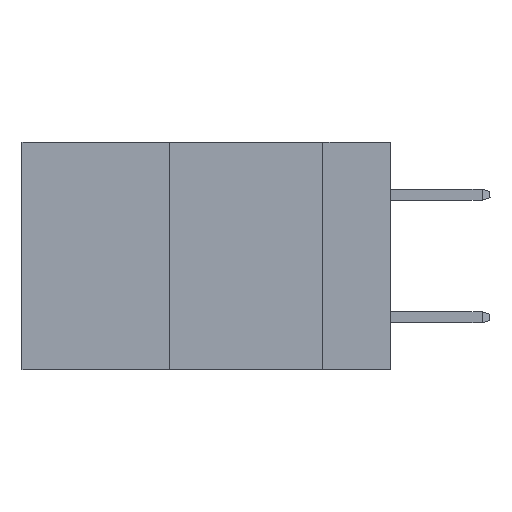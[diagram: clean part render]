
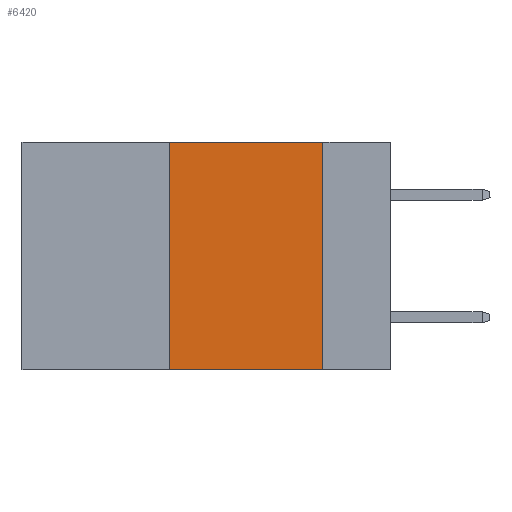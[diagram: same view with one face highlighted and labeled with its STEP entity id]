
A CAD part, left-side view. The second image highlights one B-rep face of the part: STEP entity #6420.
In plain terms, the highlighted planar face has unit normal (-1, 0, 0).
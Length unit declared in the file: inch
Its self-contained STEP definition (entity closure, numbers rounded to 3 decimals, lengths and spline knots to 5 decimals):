
#616 = CARTESIAN_POINT ( 'NONE',  ( 0., 0.6, 0. ) ) ;
#1344 = VECTOR ( 'NONE', #9300, 39.37008 ) ;
#1706 = DIRECTION ( 'NONE',  ( 0., 0., -1. ) ) ;
#1831 = CARTESIAN_POINT ( 'NONE',  ( 0., 0.11, 0. ) ) ;
#1977 = DIRECTION ( 'NONE',  ( 0., 0., -1. ) ) ;
#2207 = EDGE_CURVE ( 'NONE', #10146, #8205, #5850, .T. ) ;
#3096 = EDGE_CURVE ( 'NONE', #8205, #6480, #4719, .T. ) ;
#3157 = ORIENTED_EDGE ( 'NONE', *, *, #2207, .F. ) ;
#4719 = LINE ( 'NONE', #7437, #6367 ) ;
#5142 = ORIENTED_EDGE ( 'NONE', *, *, #13858, .T. ) ;
#5850 = LINE ( 'NONE', #616, #12321 ) ;
#6367 = VECTOR ( 'NONE', #1706, 39.37008 ) ;
#6420 = ADVANCED_FACE ( 'NONE', ( #14247 ), #9976, .F. ) ;
#6480 = VERTEX_POINT ( 'NONE', #14125 ) ;
#7437 = CARTESIAN_POINT ( 'NONE',  ( 0., 0.11, 0. ) ) ;
#8205 = VERTEX_POINT ( 'NONE', #1831 ) ;
#8292 = ORIENTED_EDGE ( 'NONE', *, *, #8927, .F. ) ;
#8363 = CARTESIAN_POINT ( 'NONE',  ( 0., 0.36, 0. ) ) ;
#8927 = EDGE_CURVE ( 'NONE', #10553, #10146, #13798, .T. ) ;
#9061 = EDGE_LOOP ( 'NONE', ( #10033, #3157, #8292, #5142 ) ) ;
#9300 = DIRECTION ( 'NONE',  ( 0., 0., 1. ) ) ;
#9951 = DIRECTION ( 'NONE',  ( 0., -1., 0. ) ) ;
#9976 = PLANE ( 'NONE',  #10563 ) ;
#10033 = ORIENTED_EDGE ( 'NONE', *, *, #3096, .F. ) ;
#10146 = VERTEX_POINT ( 'NONE', #8363 ) ;
#10553 = VERTEX_POINT ( 'NONE', #13657 ) ;
#10563 = AXIS2_PLACEMENT_3D ( 'NONE', #10918, #12286, #1977 ) ;
#10868 = CARTESIAN_POINT ( 'NONE',  ( 0., 0.36, 0. ) ) ;
#10918 = CARTESIAN_POINT ( 'NONE',  ( 0., 0.6, 0. ) ) ;
#11051 = DIRECTION ( 'NONE',  ( 0., -1., 0. ) ) ;
#11470 = LINE ( 'NONE', #12259, #14710 ) ;
#12259 = CARTESIAN_POINT ( 'NONE',  ( 0., 0.6, -0.37 ) ) ;
#12286 = DIRECTION ( 'NONE',  ( 1., 0., 0. ) ) ;
#12321 = VECTOR ( 'NONE', #11051, 39.37008 ) ;
#13657 = CARTESIAN_POINT ( 'NONE',  ( 0., 0.36, -0.37 ) ) ;
#13798 = LINE ( 'NONE', #10868, #1344 ) ;
#13858 = EDGE_CURVE ( 'NONE', #10553, #6480, #11470, .T. ) ;
#14125 = CARTESIAN_POINT ( 'NONE',  ( 0., 0.11, -0.37 ) ) ;
#14247 = FACE_OUTER_BOUND ( 'NONE', #9061, .T. ) ;
#14710 = VECTOR ( 'NONE', #9951, 39.37008 ) ;
